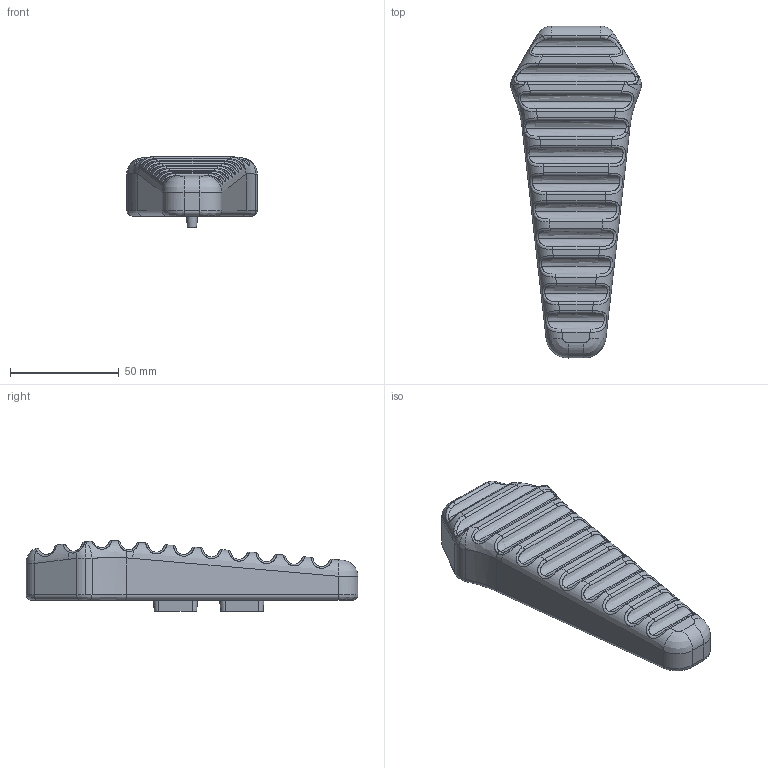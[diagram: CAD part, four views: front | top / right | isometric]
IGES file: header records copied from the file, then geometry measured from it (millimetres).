
Start section: SolidWorks IGES file using analytic representation for surfaces
Global section: file name: Stock body 3.IGS; native system: SolidWorks 2012; preprocessor: SolidWorks 2012; author: Pld; date: 131010.171239; units: inch
Bounding box: 59.93 x 152.4 x 32.33 mm (x, y, z)
Surface area: 20940.1 mm2 (no closed solid volume)
Topology: 0 solids, 0 shells, 152 faces, 1675 edges, 1675 vertices
Faces by surface type: revolution 79, bspline 73
